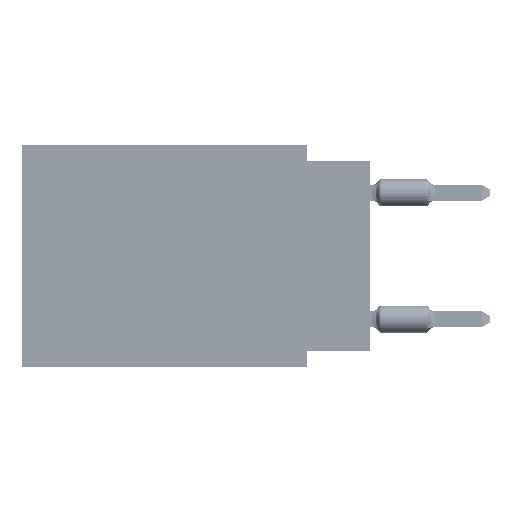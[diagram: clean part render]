
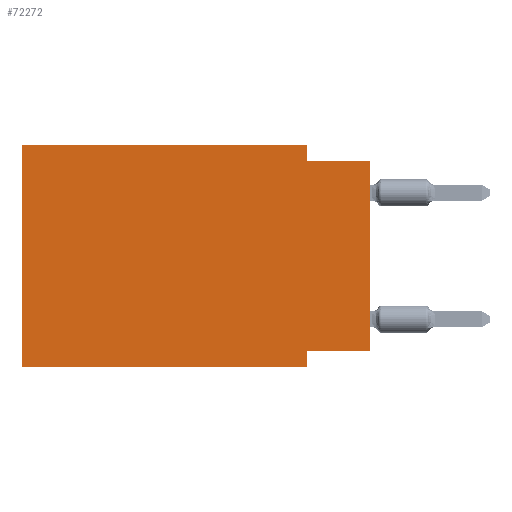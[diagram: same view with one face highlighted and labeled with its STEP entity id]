
A CAD part, left-side view. The second image highlights one B-rep face of the part: STEP entity #72272.
In plain terms, the highlighted planar face has unit normal (-1, 0, 0).
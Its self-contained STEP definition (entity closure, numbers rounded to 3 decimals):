
#372 = VERTEX_POINT ( 'NONE', #5020 ) ;
#1940 = CARTESIAN_POINT ( 'NONE',  ( 0., 2.54, -0.635 ) ) ;
#3545 = VERTEX_POINT ( 'NONE', #71562 ) ;
#3657 = ORIENTED_EDGE ( 'NONE', *, *, #22910, .F. ) ;
#5020 = CARTESIAN_POINT ( 'NONE',  ( 0., 0., -0.635 ) ) ;
#5529 = EDGE_CURVE ( 'NONE', #3545, #372, #70847, .T. ) ;
#9087 = CARTESIAN_POINT ( 'NONE',  ( 0., 13.97, 0. ) ) ;
#11485 = VERTEX_POINT ( 'NONE', #9087 ) ;
#15780 = CARTESIAN_POINT ( 'NONE',  ( 0., 2.54, -8.255 ) ) ;
#18122 = ORIENTED_EDGE ( 'NONE', *, *, #21762, .F. ) ;
#19018 = LINE ( 'NONE', #88326, #25455 ) ;
#19860 = LINE ( 'NONE', #58786, #68225 ) ;
#20145 = EDGE_CURVE ( 'NONE', #21952, #85590, #19860, .T. ) ;
#21762 = EDGE_CURVE ( 'NONE', #54831, #42737, #40270, .T. ) ;
#21952 = VERTEX_POINT ( 'NONE', #22487 ) ;
#21958 = VECTOR ( 'NONE', #24304, 1000. ) ;
#22361 = VECTOR ( 'NONE', #36954, 1000. ) ;
#22487 = CARTESIAN_POINT ( 'NONE',  ( 0., 13.97, -8.89 ) ) ;
#22910 = EDGE_CURVE ( 'NONE', #3545, #76652, #63675, .T. ) ;
#24304 = DIRECTION ( 'NONE',  ( 0., 0., 1. ) ) ;
#25455 = VECTOR ( 'NONE', #57954, 1000. ) ;
#26598 = DIRECTION ( 'NONE',  ( 0., 0., -1. ) ) ;
#29637 = LINE ( 'NONE', #91866, #58185 ) ;
#29976 = DIRECTION ( 'NONE',  ( 0., 0., 1. ) ) ;
#30476 = CARTESIAN_POINT ( 'NONE',  ( 0., 13.97, 0. ) ) ;
#34870 = EDGE_LOOP ( 'NONE', ( #51994, #38322, #18122, #98428, #99425, #86076, #36067, #3657 ) ) ;
#36067 = ORIENTED_EDGE ( 'NONE', *, *, #94073, .F. ) ;
#36954 = DIRECTION ( 'NONE',  ( 0., -1., 0. ) ) ;
#38322 = ORIENTED_EDGE ( 'NONE', *, *, #79106, .F. ) ;
#39696 = DIRECTION ( 'NONE',  ( 0., 0., -1. ) ) ;
#40270 = LINE ( 'NONE', #71144, #52254 ) ;
#41178 = FACE_OUTER_BOUND ( 'NONE', #34870, .T. ) ;
#42737 = VERTEX_POINT ( 'NONE', #1940 ) ;
#46506 = CARTESIAN_POINT ( 'NONE',  ( 0., 0., -8.255 ) ) ;
#47493 = DIRECTION ( 'NONE',  ( 0., 1., 0. ) ) ;
#47781 = DIRECTION ( 'NONE',  ( 1., 0., 0. ) ) ;
#50698 = DIRECTION ( 'NONE',  ( 0., -1., 0. ) ) ;
#51994 = ORIENTED_EDGE ( 'NONE', *, *, #5529, .T. ) ;
#52254 = VECTOR ( 'NONE', #26598, 1000. ) ;
#54831 = VERTEX_POINT ( 'NONE', #95370 ) ;
#57721 = LINE ( 'NONE', #83494, #22361 ) ;
#57954 = DIRECTION ( 'NONE',  ( 0., 0., -1. ) ) ;
#58185 = VECTOR ( 'NONE', #99455, 1000. ) ;
#58786 = CARTESIAN_POINT ( 'NONE',  ( 0., 13.97, -8.89 ) ) ;
#63675 = LINE ( 'NONE', #46506, #73429 ) ;
#68225 = VECTOR ( 'NONE', #50698, 1000. ) ;
#70527 = VECTOR ( 'NONE', #29976, 1000. ) ;
#70847 = LINE ( 'NONE', #78436, #21958 ) ;
#71144 = CARTESIAN_POINT ( 'NONE',  ( 0., 2.54, 0. ) ) ;
#71562 = CARTESIAN_POINT ( 'NONE',  ( 0., 0., -8.255 ) ) ;
#72087 = AXIS2_PLACEMENT_3D ( 'NONE', #87720, #47781, #39696 ) ;
#72272 = ADVANCED_FACE ( 'NONE', ( #41178 ), #79148, .F. ) ;
#73429 = VECTOR ( 'NONE', #47493, 1000. ) ;
#75184 = CARTESIAN_POINT ( 'NONE',  ( 0., 2.54, -8.89 ) ) ;
#76652 = VERTEX_POINT ( 'NONE', #15780 ) ;
#78436 = CARTESIAN_POINT ( 'NONE',  ( 0., 0., 0. ) ) ;
#79106 = EDGE_CURVE ( 'NONE', #42737, #372, #29637, .T. ) ;
#79148 = PLANE ( 'NONE',  #72087 ) ;
#83494 = CARTESIAN_POINT ( 'NONE',  ( 0., 13.97, 0. ) ) ;
#85590 = VERTEX_POINT ( 'NONE', #75184 ) ;
#86076 = ORIENTED_EDGE ( 'NONE', *, *, #20145, .T. ) ;
#87720 = CARTESIAN_POINT ( 'NONE',  ( 0., 13.97, 0. ) ) ;
#88326 = CARTESIAN_POINT ( 'NONE',  ( 0., 2.54, -8.89 ) ) ;
#91866 = CARTESIAN_POINT ( 'NONE',  ( 0., 0., -0.635 ) ) ;
#93346 = EDGE_CURVE ( 'NONE', #21952, #11485, #99291, .T. ) ;
#94073 = EDGE_CURVE ( 'NONE', #76652, #85590, #19018, .T. ) ;
#94961 = EDGE_CURVE ( 'NONE', #11485, #54831, #57721, .T. ) ;
#95370 = CARTESIAN_POINT ( 'NONE',  ( 0., 2.54, 0. ) ) ;
#98428 = ORIENTED_EDGE ( 'NONE', *, *, #94961, .F. ) ;
#99291 = LINE ( 'NONE', #30476, #70527 ) ;
#99425 = ORIENTED_EDGE ( 'NONE', *, *, #93346, .F. ) ;
#99455 = DIRECTION ( 'NONE',  ( 0., -1., 0. ) ) ;
